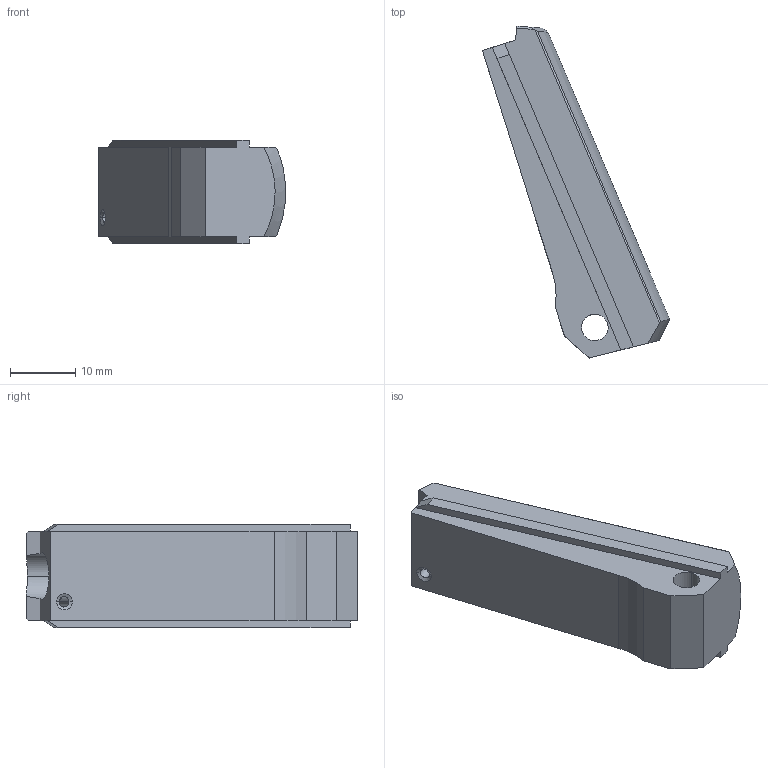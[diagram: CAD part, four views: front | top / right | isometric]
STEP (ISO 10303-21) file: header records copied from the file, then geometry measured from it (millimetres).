
FILE_DESCRIPTION((''),'2;1');
FILE_NAME('MSBR-13_1_1_1_1_1','2023-06-18T',('WILLIAM'),(''),'CREO PARAMETRIC BY PTC INC, 2014500','CREO PARAMETRIC BY PTC INC, 2014500','');
FILE_SCHEMA(('CONFIG_CONTROL_DESIGN'));
Length unit declared in the file: millimetre
Products named in the file (1): MSBR-13_1_1_1_1_1
Bounding box: 28.6 x 50.7 x 15.8 mm (x, y, z)
Volume: 6792.4 mm3; surface area: 4204.4 mm2
Topology: 1 solids, 1 shells, 40 faces, 111 edges, 72 vertices
Faces by surface type: plane 26, cylinder 8, cone 4, bspline 2
Entity records: 1560 total; most frequent: CARTESIAN_POINT 530, ORIENTED_EDGE 222, DIRECTION 173, EDGE_CURVE 111, VERTEX_POINT 72, VECTOR 69, LINE 69, AXIS2_PLACEMENT_3D 52
